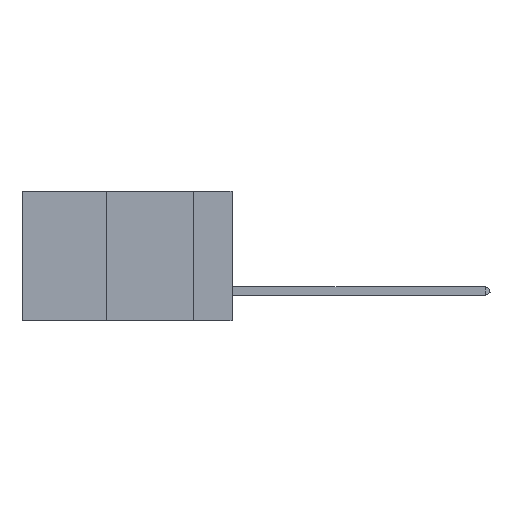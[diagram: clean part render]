
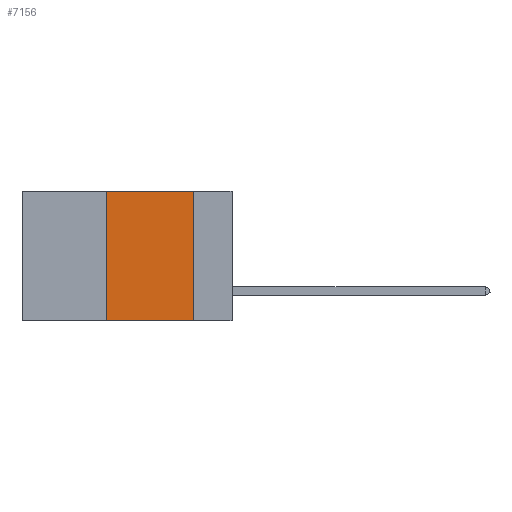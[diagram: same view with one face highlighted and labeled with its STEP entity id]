
A CAD part, left-side view. The second image highlights one B-rep face of the part: STEP entity #7156.
In plain terms, the highlighted planar face has unit normal (-1, 0, 0).
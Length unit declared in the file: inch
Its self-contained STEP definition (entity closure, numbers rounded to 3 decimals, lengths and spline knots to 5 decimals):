
#120 = CARTESIAN_POINT ( 'NONE',  ( 0., 0.11, 0. ) ) ;
#3161 = CARTESIAN_POINT ( 'NONE',  ( 0., 0.36, -0.37 ) ) ;
#3232 = VECTOR ( 'NONE', #45798, 39.37008 ) ;
#6748 = DIRECTION ( 'NONE',  ( 1., 0., 0. ) ) ;
#6872 = LINE ( 'NONE', #19585, #24726 ) ;
#7156 = ADVANCED_FACE ( 'NONE', ( #42816 ), #42283, .F. ) ;
#8433 = LINE ( 'NONE', #27551, #17341 ) ;
#9625 = ORIENTED_EDGE ( 'NONE', *, *, #15514, .F. ) ;
#10622 = CARTESIAN_POINT ( 'NONE',  ( 0., 0.6, -0.37 ) ) ;
#10708 = VERTEX_POINT ( 'NONE', #34753 ) ;
#10908 = VERTEX_POINT ( 'NONE', #3161 ) ;
#13384 = LINE ( 'NONE', #10622, #44216 ) ;
#15514 = EDGE_CURVE ( 'NONE', #21779, #21324, #45807, .T. ) ;
#16508 = CARTESIAN_POINT ( 'NONE',  ( 0., 0.36, 0. ) ) ;
#17341 = VECTOR ( 'NONE', #34606, 39.37008 ) ;
#19585 = CARTESIAN_POINT ( 'NONE',  ( 0., 0.36, 0. ) ) ;
#21081 = CARTESIAN_POINT ( 'NONE',  ( 0., 0.6, 0. ) ) ;
#21324 = VERTEX_POINT ( 'NONE', #120 ) ;
#21779 = VERTEX_POINT ( 'NONE', #16508 ) ;
#21973 = ORIENTED_EDGE ( 'NONE', *, *, #28728, .F. ) ;
#22055 = ORIENTED_EDGE ( 'NONE', *, *, #41778, .F. ) ;
#24726 = VECTOR ( 'NONE', #34622, 39.37008 ) ;
#27551 = CARTESIAN_POINT ( 'NONE',  ( 0., 0.11, 0. ) ) ;
#28547 = DIRECTION ( 'NONE',  ( 0., -1., 0. ) ) ;
#28728 = EDGE_CURVE ( 'NONE', #10908, #21779, #6872, .T. ) ;
#31640 = EDGE_CURVE ( 'NONE', #10908, #10708, #13384, .T. ) ;
#34479 = ORIENTED_EDGE ( 'NONE', *, *, #31640, .T. ) ;
#34606 = DIRECTION ( 'NONE',  ( 0., 0., -1. ) ) ;
#34622 = DIRECTION ( 'NONE',  ( 0., 0., 1. ) ) ;
#34753 = CARTESIAN_POINT ( 'NONE',  ( 0., 0.11, -0.37 ) ) ;
#38533 = DIRECTION ( 'NONE',  ( 0., 0., -1. ) ) ;
#41439 = AXIS2_PLACEMENT_3D ( 'NONE', #21081, #6748, #38533 ) ;
#41778 = EDGE_CURVE ( 'NONE', #21324, #10708, #8433, .T. ) ;
#42202 = CARTESIAN_POINT ( 'NONE',  ( 0., 0.6, 0. ) ) ;
#42283 = PLANE ( 'NONE',  #41439 ) ;
#42816 = FACE_OUTER_BOUND ( 'NONE', #43630, .T. ) ;
#43630 = EDGE_LOOP ( 'NONE', ( #22055, #9625, #21973, #34479 ) ) ;
#44216 = VECTOR ( 'NONE', #28547, 39.37008 ) ;
#45798 = DIRECTION ( 'NONE',  ( 0., -1., 0. ) ) ;
#45807 = LINE ( 'NONE', #42202, #3232 ) ;
